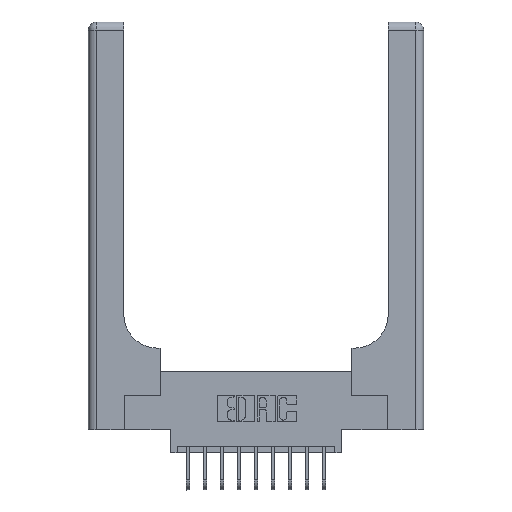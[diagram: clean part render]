
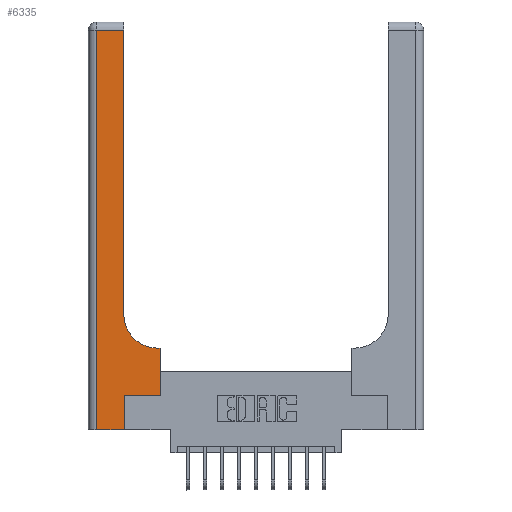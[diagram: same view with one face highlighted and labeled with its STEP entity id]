
A CAD part, top view. The second image highlights one B-rep face of the part: STEP entity #6335.
In plain terms, the highlighted planar face has unit normal (0, 0, 1).
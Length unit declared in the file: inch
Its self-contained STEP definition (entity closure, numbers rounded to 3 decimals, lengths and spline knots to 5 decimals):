
#442 = CARTESIAN_POINT ( 'NONE',  ( 0.06, 2.94, 0.37 ) ) ;
#715 = CARTESIAN_POINT ( 'NONE',  ( 0.51, 0.6, 0.37 ) ) ;
#811 = ORIENTED_EDGE ( 'NONE', *, *, #9455, .T. ) ;
#946 = DIRECTION ( 'NONE',  ( 1., 0., 0. ) ) ;
#1057 = CARTESIAN_POINT ( 'NONE',  ( 0.06, 0., 0.37 ) ) ;
#1253 = ORIENTED_EDGE ( 'NONE', *, *, #3670, .T. ) ;
#1327 = DIRECTION ( 'NONE',  ( 0., 0., -1. ) ) ;
#1913 = VERTEX_POINT ( 'NONE', #9604 ) ;
#1975 = LINE ( 'NONE', #6930, #13910 ) ;
#2028 = DIRECTION ( 'NONE',  ( 1., 0., 0. ) ) ;
#2349 = VERTEX_POINT ( 'NONE', #715 ) ;
#2376 = CARTESIAN_POINT ( 'NONE',  ( 0.528, 0.25, 0.37 ) ) ;
#2458 = VERTEX_POINT ( 'NONE', #5681 ) ;
#2644 = LINE ( 'NONE', #6798, #8691 ) ;
#2787 = AXIS2_PLACEMENT_3D ( 'NONE', #8549, #1327, #9760 ) ;
#3090 = DIRECTION ( 'NONE',  ( 0., 0., -1. ) ) ;
#3359 = DIRECTION ( 'NONE',  ( -1., 0., 0. ) ) ;
#3670 = EDGE_CURVE ( 'NONE', #2349, #8868, #6676, .T. ) ;
#3811 = EDGE_CURVE ( 'NONE', #3875, #2458, #1975, .T. ) ;
#3829 = EDGE_CURVE ( 'NONE', #11559, #2349, #10820, .T. ) ;
#3875 = VERTEX_POINT ( 'NONE', #1057 ) ;
#4245 = DIRECTION ( 'NONE',  ( -1., 0., 0. ) ) ;
#4368 = ORIENTED_EDGE ( 'NONE', *, *, #7124, .T. ) ;
#4383 = CARTESIAN_POINT ( 'NONE',  ( 0.265, 0.25, 0.37 ) ) ;
#4410 = VECTOR ( 'NONE', #3359, 39.37008 ) ;
#4431 = DIRECTION ( 'NONE',  ( 0., 1., 0. ) ) ;
#4768 = ORIENTED_EDGE ( 'NONE', *, *, #9912, .T. ) ;
#4776 = VECTOR ( 'NONE', #11734, 39.37008 ) ;
#5089 = VERTEX_POINT ( 'NONE', #13961 ) ;
#5356 = ORIENTED_EDGE ( 'NONE', *, *, #3811, .T. ) ;
#5464 = ORIENTED_EDGE ( 'NONE', *, *, #6072, .T. ) ;
#5557 = ORIENTED_EDGE ( 'NONE', *, *, #9340, .T. ) ;
#5681 = CARTESIAN_POINT ( 'NONE',  ( 0.265, 0., 0.37 ) ) ;
#6072 = EDGE_CURVE ( 'NONE', #8756, #3875, #6598, .T. ) ;
#6270 = AXIS2_PLACEMENT_3D ( 'NONE', #10316, #3090, #11472 ) ;
#6335 = ADVANCED_FACE ( 'NONE', ( #9650 ), #9658, .F. ) ;
#6588 = CARTESIAN_POINT ( 'NONE',  ( 0.26, 0.85, 0.37 ) ) ;
#6598 = LINE ( 'NONE', #10325, #12205 ) ;
#6676 = CIRCLE ( 'NONE', #6270, 0.25 ) ;
#6684 = CARTESIAN_POINT ( 'NONE',  ( 0.528, 0.6, 0.37 ) ) ;
#6798 = CARTESIAN_POINT ( 'NONE',  ( 0.265, 0., 0.37 ) ) ;
#6930 = CARTESIAN_POINT ( 'NONE',  ( 0., 0., 0.37 ) ) ;
#7124 = EDGE_CURVE ( 'NONE', #2458, #11774, #2644, .T. ) ;
#8156 = CARTESIAN_POINT ( 'NONE',  ( 0.26, 0.6, 0.37 ) ) ;
#8359 = LINE ( 'NONE', #4383, #11494 ) ;
#8549 = CARTESIAN_POINT ( 'NONE',  ( 0., 3., 0.37 ) ) ;
#8691 = VECTOR ( 'NONE', #4431, 39.37008 ) ;
#8756 = VERTEX_POINT ( 'NONE', #442 ) ;
#8868 = VERTEX_POINT ( 'NONE', #6588 ) ;
#9340 = EDGE_CURVE ( 'NONE', #5089, #8756, #9891, .T. ) ;
#9455 = EDGE_CURVE ( 'NONE', #8868, #5089, #11508, .T. ) ;
#9604 = CARTESIAN_POINT ( 'NONE',  ( 0.528, 0.25, 0.37 ) ) ;
#9650 = FACE_OUTER_BOUND ( 'NONE', #12135, .T. ) ;
#9658 = PLANE ( 'NONE',  #2787 ) ;
#9673 = CARTESIAN_POINT ( 'NONE',  ( 0.265, 0.25, 0.37 ) ) ;
#9760 = DIRECTION ( 'NONE',  ( -1., 0., 0. ) ) ;
#9891 = LINE ( 'NONE', #10261, #15360 ) ;
#9912 = EDGE_CURVE ( 'NONE', #11774, #1913, #8359, .T. ) ;
#10261 = CARTESIAN_POINT ( 'NONE',  ( 0., 2.94, 0.37 ) ) ;
#10316 = CARTESIAN_POINT ( 'NONE',  ( 0.51, 0.85, 0.37 ) ) ;
#10325 = CARTESIAN_POINT ( 'NONE',  ( 0.06, 3., 0.37 ) ) ;
#10563 = CARTESIAN_POINT ( 'NONE',  ( 0.26, 3., 0.37 ) ) ;
#10652 = LINE ( 'NONE', #2376, #13748 ) ;
#10781 = DIRECTION ( 'NONE',  ( 0., 1., 0. ) ) ;
#10820 = LINE ( 'NONE', #8156, #4410 ) ;
#11472 = DIRECTION ( 'NONE',  ( 1., 0., 0. ) ) ;
#11494 = VECTOR ( 'NONE', #2028, 39.37008 ) ;
#11508 = LINE ( 'NONE', #10563, #4776 ) ;
#11559 = VERTEX_POINT ( 'NONE', #6684 ) ;
#11734 = DIRECTION ( 'NONE',  ( 0., 1., 0. ) ) ;
#11774 = VERTEX_POINT ( 'NONE', #9673 ) ;
#11818 = ORIENTED_EDGE ( 'NONE', *, *, #3829, .T. ) ;
#12135 = EDGE_LOOP ( 'NONE', ( #811, #5557, #5464, #5356, #4368, #4768, #14506, #11818, #1253 ) ) ;
#12205 = VECTOR ( 'NONE', #12666, 39.37008 ) ;
#12666 = DIRECTION ( 'NONE',  ( 0., -1., 0. ) ) ;
#13748 = VECTOR ( 'NONE', #10781, 39.37008 ) ;
#13910 = VECTOR ( 'NONE', #946, 39.37008 ) ;
#13961 = CARTESIAN_POINT ( 'NONE',  ( 0.26, 2.94, 0.37 ) ) ;
#14506 = ORIENTED_EDGE ( 'NONE', *, *, #15143, .T. ) ;
#15143 = EDGE_CURVE ( 'NONE', #1913, #11559, #10652, .T. ) ;
#15360 = VECTOR ( 'NONE', #4245, 39.37008 ) ;
